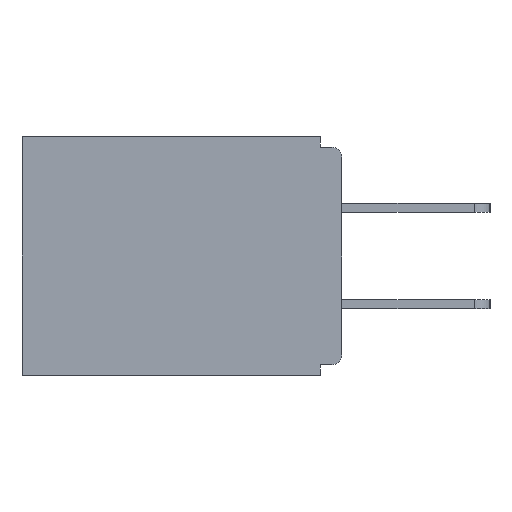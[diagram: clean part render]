
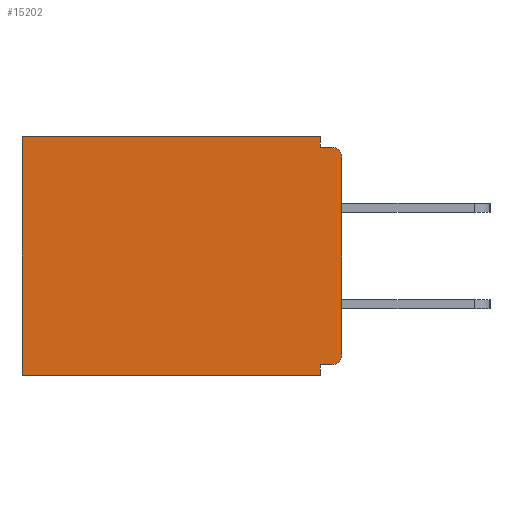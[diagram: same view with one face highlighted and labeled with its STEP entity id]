
A CAD part, left-side view. The second image highlights one B-rep face of the part: STEP entity #15202.
In plain terms, the highlighted planar face has unit normal (-1, 0, 0).
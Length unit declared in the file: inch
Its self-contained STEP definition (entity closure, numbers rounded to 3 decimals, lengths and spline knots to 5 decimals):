
#69 = CARTESIAN_POINT ( 'NONE',  ( 0.298, 0.031, -0.343 ) ) ;
#142 = EDGE_CURVE ( 'NONE', #19461, #6964, #19072, .T. ) ;
#562 = CIRCLE ( 'NONE', #6076, 0.015 ) ;
#662 = VERTEX_POINT ( 'NONE', #2250 ) ;
#737 = VECTOR ( 'NONE', #14242, 39.37008 ) ;
#773 = EDGE_CURVE ( 'NONE', #17229, #19461, #12446, .T. ) ;
#1271 = VECTOR ( 'NONE', #18380, 39.37008 ) ;
#1476 = CARTESIAN_POINT ( 'NONE',  ( 0.298, 0., 0. ) ) ;
#1710 = ORIENTED_EDGE ( 'NONE', *, *, #6954, .F. ) ;
#2228 = ORIENTED_EDGE ( 'NONE', *, *, #4122, .F. ) ;
#2250 = CARTESIAN_POINT ( 'NONE',  ( 0.298, 0.015, -0.015 ) ) ;
#2566 = VERTEX_POINT ( 'NONE', #3125 ) ;
#2805 = CARTESIAN_POINT ( 'NONE',  ( 0.298, 0., -0.328 ) ) ;
#2886 = CARTESIAN_POINT ( 'NONE',  ( 0.298, 0.031, -0.015 ) ) ;
#2959 = LINE ( 'NONE', #69, #8312 ) ;
#3003 = LINE ( 'NONE', #18595, #18799 ) ;
#3125 = CARTESIAN_POINT ( 'NONE',  ( 0.298, 0.015, -0.328 ) ) ;
#3292 = CARTESIAN_POINT ( 'NONE',  ( 0.298, 0.015, -0.03 ) ) ;
#3760 = PLANE ( 'NONE',  #4422 ) ;
#3850 = CIRCLE ( 'NONE', #7578, 0.015 ) ;
#3900 = DIRECTION ( 'NONE',  ( 1., 0., 0. ) ) ;
#4122 = EDGE_CURVE ( 'NONE', #16051, #11492, #5165, .T. ) ;
#4422 = AXIS2_PLACEMENT_3D ( 'NONE', #13695, #3900, #16875 ) ;
#4505 = CARTESIAN_POINT ( 'NONE',  ( 0.298, 0., -0.03 ) ) ;
#5165 = LINE ( 'NONE', #1476, #18389 ) ;
#5826 = EDGE_CURVE ( 'NONE', #16901, #7277, #12471, .T. ) ;
#5991 = VECTOR ( 'NONE', #11519, 39.37008 ) ;
#6076 = AXIS2_PLACEMENT_3D ( 'NONE', #3292, #12863, #6312 ) ;
#6312 = DIRECTION ( 'NONE',  ( 0., 0., -1. ) ) ;
#6563 = DIRECTION ( 'NONE',  ( 0., 1., 0. ) ) ;
#6954 = EDGE_CURVE ( 'NONE', #17229, #14477, #2959, .T. ) ;
#6964 = VERTEX_POINT ( 'NONE', #16283 ) ;
#7277 = VERTEX_POINT ( 'NONE', #19373 ) ;
#7420 = FACE_OUTER_BOUND ( 'NONE', #10776, .T. ) ;
#7578 = AXIS2_PLACEMENT_3D ( 'NONE', #17333, #18950, #11124 ) ;
#7883 = CARTESIAN_POINT ( 'NONE',  ( 0.298, 0.46, 0. ) ) ;
#8225 = DIRECTION ( 'NONE',  ( 0., 0., -1. ) ) ;
#8312 = VECTOR ( 'NONE', #8225, 39.37008 ) ;
#8854 = DIRECTION ( 'NONE',  ( 0., 1., 0. ) ) ;
#9087 = EDGE_CURVE ( 'NONE', #16051, #662, #562, .T. ) ;
#9562 = CARTESIAN_POINT ( 'NONE',  ( 0.298, 0.031, -0.343 ) ) ;
#9879 = CARTESIAN_POINT ( 'NONE',  ( 0.298, 0., -0.015 ) ) ;
#10776 = EDGE_LOOP ( 'NONE', ( #18856, #12304, #1710, #12666, #13769, #14843, #19336, #19702, #15696, #2228 ) ) ;
#11124 = DIRECTION ( 'NONE',  ( 0., 0., -1. ) ) ;
#11484 = EDGE_CURVE ( 'NONE', #7277, #6964, #3003, .T. ) ;
#11492 = VERTEX_POINT ( 'NONE', #18390 ) ;
#11519 = DIRECTION ( 'NONE',  ( 0., -1., 0. ) ) ;
#12304 = ORIENTED_EDGE ( 'NONE', *, *, #19610, .F. ) ;
#12446 = LINE ( 'NONE', #13049, #19807 ) ;
#12471 = LINE ( 'NONE', #9562, #19832 ) ;
#12666 = ORIENTED_EDGE ( 'NONE', *, *, #773, .T. ) ;
#12693 = LINE ( 'NONE', #2805, #737 ) ;
#12724 = DIRECTION ( 'NONE',  ( 0., 0., -1. ) ) ;
#12863 = DIRECTION ( 'NONE',  ( -1., 0., 0. ) ) ;
#13049 = CARTESIAN_POINT ( 'NONE',  ( 0.298, 0., 0. ) ) ;
#13695 = CARTESIAN_POINT ( 'NONE',  ( 0.298, 0., 0. ) ) ;
#13769 = ORIENTED_EDGE ( 'NONE', *, *, #142, .T. ) ;
#14110 = CARTESIAN_POINT ( 'NONE',  ( 0.298, 0.031, 0. ) ) ;
#14242 = DIRECTION ( 'NONE',  ( 0., 1., 0. ) ) ;
#14477 = VERTEX_POINT ( 'NONE', #2886 ) ;
#14843 = ORIENTED_EDGE ( 'NONE', *, *, #11484, .F. ) ;
#15202 = ADVANCED_FACE ( 'NONE', ( #7420 ), #3760, .F. ) ;
#15696 = ORIENTED_EDGE ( 'NONE', *, *, #15972, .T. ) ;
#15740 = CARTESIAN_POINT ( 'NONE',  ( 0.298, 0.031, -0.328 ) ) ;
#15972 = EDGE_CURVE ( 'NONE', #2566, #11492, #3850, .T. ) ;
#16051 = VERTEX_POINT ( 'NONE', #4505 ) ;
#16283 = CARTESIAN_POINT ( 'NONE',  ( 0.298, 0.46, -0.343 ) ) ;
#16545 = CARTESIAN_POINT ( 'NONE',  ( 0.298, 0.46, 0. ) ) ;
#16875 = DIRECTION ( 'NONE',  ( 0., 0., -1. ) ) ;
#16901 = VERTEX_POINT ( 'NONE', #15740 ) ;
#17229 = VERTEX_POINT ( 'NONE', #14110 ) ;
#17333 = CARTESIAN_POINT ( 'NONE',  ( 0.298, 0.015, -0.313 ) ) ;
#17384 = EDGE_CURVE ( 'NONE', #2566, #16901, #12693, .T. ) ;
#18380 = DIRECTION ( 'NONE',  ( 0., 0., -1. ) ) ;
#18389 = VECTOR ( 'NONE', #12724, 39.37008 ) ;
#18390 = CARTESIAN_POINT ( 'NONE',  ( 0.298, 0., -0.313 ) ) ;
#18595 = CARTESIAN_POINT ( 'NONE',  ( 0.298, 0., -0.343 ) ) ;
#18704 = DIRECTION ( 'NONE',  ( 0., 0., -1. ) ) ;
#18799 = VECTOR ( 'NONE', #8854, 39.37008 ) ;
#18856 = ORIENTED_EDGE ( 'NONE', *, *, #9087, .T. ) ;
#18950 = DIRECTION ( 'NONE',  ( -1., 0., 0. ) ) ;
#19072 = LINE ( 'NONE', #16545, #1271 ) ;
#19336 = ORIENTED_EDGE ( 'NONE', *, *, #5826, .F. ) ;
#19373 = CARTESIAN_POINT ( 'NONE',  ( 0.298, 0.031, -0.343 ) ) ;
#19458 = LINE ( 'NONE', #9879, #5991 ) ;
#19461 = VERTEX_POINT ( 'NONE', #7883 ) ;
#19610 = EDGE_CURVE ( 'NONE', #14477, #662, #19458, .T. ) ;
#19702 = ORIENTED_EDGE ( 'NONE', *, *, #17384, .F. ) ;
#19807 = VECTOR ( 'NONE', #6563, 39.37008 ) ;
#19832 = VECTOR ( 'NONE', #18704, 39.37008 ) ;
